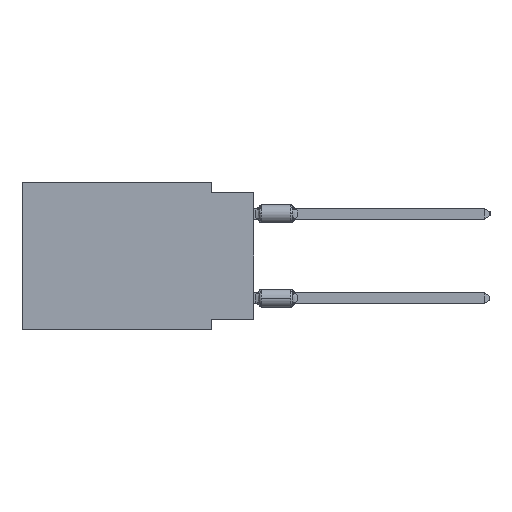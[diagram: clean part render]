
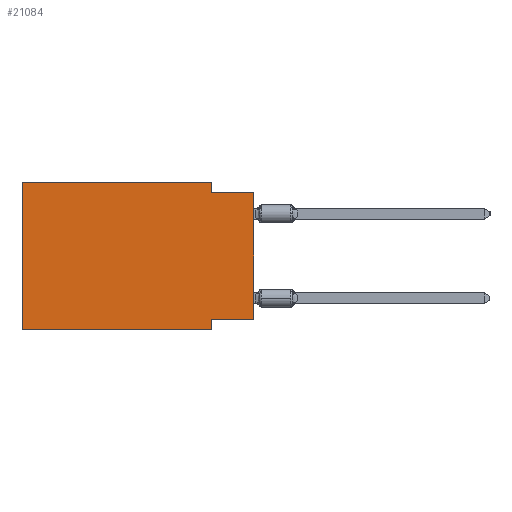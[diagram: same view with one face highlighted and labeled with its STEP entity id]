
A CAD part, left-side view. The second image highlights one B-rep face of the part: STEP entity #21084.
In plain terms, the highlighted planar face has unit normal (-1, 0, 0).
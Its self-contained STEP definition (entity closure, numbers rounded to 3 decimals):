
#956 = PLANE ( 'NONE',  #33208 ) ;
#1149 = ORIENTED_EDGE ( 'NONE', *, *, #8213, .F. ) ;
#1569 = CARTESIAN_POINT ( 'NONE',  ( 0., 2.54, -8.89 ) ) ;
#2047 = CARTESIAN_POINT ( 'NONE',  ( 0., 13.97, -8.89 ) ) ;
#2264 = VECTOR ( 'NONE', #37489, 1000. ) ;
#3835 = ORIENTED_EDGE ( 'NONE', *, *, #12462, .F. ) ;
#4403 = VERTEX_POINT ( 'NONE', #17033 ) ;
#4760 = DIRECTION ( 'NONE',  ( 0., -1., 0. ) ) ;
#7417 = EDGE_LOOP ( 'NONE', ( #19287, #36715, #3835, #10148, #11746, #24275, #7582, #1149 ) ) ;
#7582 = ORIENTED_EDGE ( 'NONE', *, *, #21234, .F. ) ;
#8213 = EDGE_CURVE ( 'NONE', #17613, #34614, #35709, .T. ) ;
#8848 = CARTESIAN_POINT ( 'NONE',  ( 0., 2.54, 0. ) ) ;
#8977 = VERTEX_POINT ( 'NONE', #26439 ) ;
#9479 = EDGE_CURVE ( 'NONE', #4403, #13413, #24647, .T. ) ;
#9768 = VERTEX_POINT ( 'NONE', #23545 ) ;
#10148 = ORIENTED_EDGE ( 'NONE', *, *, #22320, .F. ) ;
#10414 = DIRECTION ( 'NONE',  ( 0., 1., 0. ) ) ;
#10605 = EDGE_CURVE ( 'NONE', #4403, #9768, #13924, .T. ) ;
#10620 = VERTEX_POINT ( 'NONE', #16850 ) ;
#10667 = DIRECTION ( 'NONE',  ( 0., 0., 1. ) ) ;
#10998 = CARTESIAN_POINT ( 'NONE',  ( 0., 13.97, 0. ) ) ;
#11179 = LINE ( 'NONE', #1569, #25211 ) ;
#11746 = ORIENTED_EDGE ( 'NONE', *, *, #10605, .F. ) ;
#12462 = EDGE_CURVE ( 'NONE', #10620, #22998, #37696, .T. ) ;
#12526 = DIRECTION ( 'NONE',  ( 0., -1., 0. ) ) ;
#13179 = CARTESIAN_POINT ( 'NONE',  ( 0., 2.54, -8.255 ) ) ;
#13413 = VERTEX_POINT ( 'NONE', #31351 ) ;
#13924 = LINE ( 'NONE', #10998, #21950 ) ;
#14399 = LINE ( 'NONE', #27197, #16348 ) ;
#16348 = VECTOR ( 'NONE', #10667, 1000. ) ;
#16850 = CARTESIAN_POINT ( 'NONE',  ( 0., 2.54, 0. ) ) ;
#17033 = CARTESIAN_POINT ( 'NONE',  ( 0., 13.97, -8.89 ) ) ;
#17454 = CARTESIAN_POINT ( 'NONE',  ( 0., 13.97, 0. ) ) ;
#17613 = VERTEX_POINT ( 'NONE', #34016 ) ;
#18465 = VECTOR ( 'NONE', #12526, 1000. ) ;
#19287 = ORIENTED_EDGE ( 'NONE', *, *, #35980, .T. ) ;
#21084 = ADVANCED_FACE ( 'NONE', ( #26477 ), #956, .F. ) ;
#21200 = CARTESIAN_POINT ( 'NONE',  ( 0., 0., -0.635 ) ) ;
#21227 = VECTOR ( 'NONE', #4760, 1000. ) ;
#21234 = EDGE_CURVE ( 'NONE', #34614, #13413, #11179, .T. ) ;
#21950 = VECTOR ( 'NONE', #23988, 1000. ) ;
#22320 = EDGE_CURVE ( 'NONE', #9768, #10620, #28432, .T. ) ;
#22998 = VERTEX_POINT ( 'NONE', #38935 ) ;
#23171 = VECTOR ( 'NONE', #10414, 1000. ) ;
#23545 = CARTESIAN_POINT ( 'NONE',  ( 0., 13.97, 0. ) ) ;
#23964 = DIRECTION ( 'NONE',  ( 0., 0., -1. ) ) ;
#23988 = DIRECTION ( 'NONE',  ( 0., 0., 1. ) ) ;
#24275 = ORIENTED_EDGE ( 'NONE', *, *, #9479, .T. ) ;
#24647 = LINE ( 'NONE', #2047, #21227 ) ;
#25211 = VECTOR ( 'NONE', #23964, 1000. ) ;
#25920 = CARTESIAN_POINT ( 'NONE',  ( 0., 0., -8.255 ) ) ;
#26439 = CARTESIAN_POINT ( 'NONE',  ( 0., 0., -0.635 ) ) ;
#26477 = FACE_OUTER_BOUND ( 'NONE', #7417, .T. ) ;
#27197 = CARTESIAN_POINT ( 'NONE',  ( 0., 0., 0. ) ) ;
#27307 = DIRECTION ( 'NONE',  ( 0., 0., -1. ) ) ;
#28110 = DIRECTION ( 'NONE',  ( 0., 0., -1. ) ) ;
#28432 = LINE ( 'NONE', #41144, #18465 ) ;
#31029 = LINE ( 'NONE', #21200, #2264 ) ;
#31351 = CARTESIAN_POINT ( 'NONE',  ( 0., 2.54, -8.89 ) ) ;
#31353 = EDGE_CURVE ( 'NONE', #22998, #8977, #31029, .T. ) ;
#33208 = AXIS2_PLACEMENT_3D ( 'NONE', #17454, #36683, #27307 ) ;
#34016 = CARTESIAN_POINT ( 'NONE',  ( 0., 0., -8.255 ) ) ;
#34614 = VERTEX_POINT ( 'NONE', #13179 ) ;
#35709 = LINE ( 'NONE', #25920, #23171 ) ;
#35980 = EDGE_CURVE ( 'NONE', #17613, #8977, #14399, .T. ) ;
#36683 = DIRECTION ( 'NONE',  ( 1., 0., 0. ) ) ;
#36715 = ORIENTED_EDGE ( 'NONE', *, *, #31353, .F. ) ;
#37489 = DIRECTION ( 'NONE',  ( 0., -1., 0. ) ) ;
#37696 = LINE ( 'NONE', #8848, #38001 ) ;
#38001 = VECTOR ( 'NONE', #28110, 1000. ) ;
#38935 = CARTESIAN_POINT ( 'NONE',  ( 0., 2.54, -0.635 ) ) ;
#41144 = CARTESIAN_POINT ( 'NONE',  ( 0., 13.97, 0. ) ) ;
